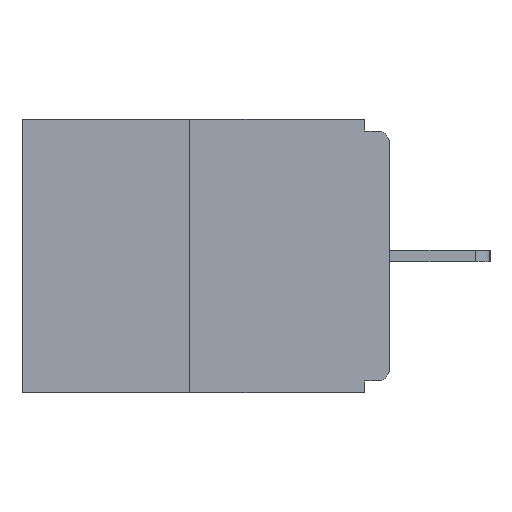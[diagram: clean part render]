
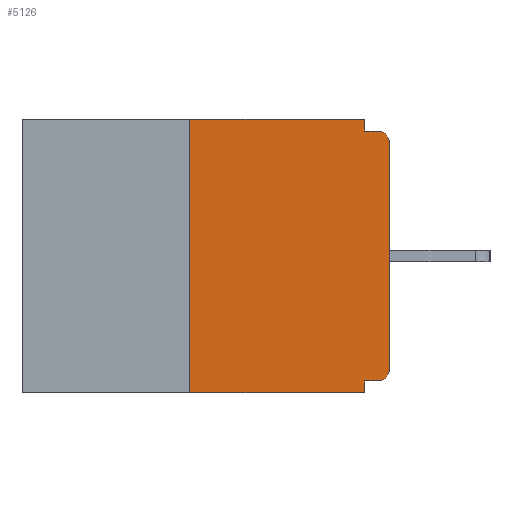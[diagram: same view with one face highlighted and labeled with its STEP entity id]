
A CAD part, left-side view. The second image highlights one B-rep face of the part: STEP entity #5126.
In plain terms, the highlighted planar face has unit normal (-1, 0, 0).
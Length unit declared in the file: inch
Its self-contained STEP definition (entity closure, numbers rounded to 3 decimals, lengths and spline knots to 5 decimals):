
#54 = CARTESIAN_POINT ( 'NONE',  ( 0., 0.031, -0.328 ) ) ;
#58 = ORIENTED_EDGE ( 'NONE', *, *, #1435, .F. ) ;
#370 = VECTOR ( 'NONE', #8513, 39.37008 ) ;
#512 = DIRECTION ( 'NONE',  ( 0., 1., 0. ) ) ;
#694 = CARTESIAN_POINT ( 'NONE',  ( 0., 0.031, -0.343 ) ) ;
#1266 = LINE ( 'NONE', #2451, #4930 ) ;
#1435 = EDGE_CURVE ( 'NONE', #9953, #11994, #3227, .T. ) ;
#1493 = DIRECTION ( 'NONE',  ( -1., 0., 0. ) ) ;
#1563 = EDGE_CURVE ( 'NONE', #3779, #13840, #5796, .T. ) ;
#2316 = DIRECTION ( 'NONE',  ( -1., 0., 0. ) ) ;
#2371 = LINE ( 'NONE', #694, #10799 ) ;
#2451 = CARTESIAN_POINT ( 'NONE',  ( 0., 0.25, 0. ) ) ;
#2717 = VERTEX_POINT ( 'NONE', #14361 ) ;
#2889 = CIRCLE ( 'NONE', #16332, 0.015 ) ;
#3047 = ORIENTED_EDGE ( 'NONE', *, *, #3152, .T. ) ;
#3152 = EDGE_CURVE ( 'NONE', #7802, #6265, #6615, .T. ) ;
#3227 = LINE ( 'NONE', #5793, #6926 ) ;
#3363 = CARTESIAN_POINT ( 'NONE',  ( 0., 0.25, 0. ) ) ;
#3403 = ORIENTED_EDGE ( 'NONE', *, *, #1563, .F. ) ;
#3779 = VERTEX_POINT ( 'NONE', #4391 ) ;
#3789 = EDGE_CURVE ( 'NONE', #8034, #10893, #13545, .T. ) ;
#3894 = CIRCLE ( 'NONE', #10600, 0.015 ) ;
#3910 = VERTEX_POINT ( 'NONE', #12890 ) ;
#4391 = CARTESIAN_POINT ( 'NONE',  ( 0., 0.015, -0.328 ) ) ;
#4912 = DIRECTION ( 'NONE',  ( 0., 0., -1. ) ) ;
#4930 = VECTOR ( 'NONE', #16602, 39.37008 ) ;
#5126 = ADVANCED_FACE ( 'NONE', ( #14626 ), #14539, .F. ) ;
#5397 = ORIENTED_EDGE ( 'NONE', *, *, #14566, .F. ) ;
#5653 = CARTESIAN_POINT ( 'NONE',  ( 0., 0.015, -0.015 ) ) ;
#5793 = CARTESIAN_POINT ( 'NONE',  ( 0., 0.46, 0. ) ) ;
#5796 = LINE ( 'NONE', #12034, #15717 ) ;
#5838 = ORIENTED_EDGE ( 'NONE', *, *, #3789, .F. ) ;
#6115 = CARTESIAN_POINT ( 'NONE',  ( 0., 0.25, -0.343 ) ) ;
#6218 = EDGE_CURVE ( 'NONE', #3779, #2717, #2889, .T. ) ;
#6265 = VERTEX_POINT ( 'NONE', #9070 ) ;
#6615 = LINE ( 'NONE', #10829, #9888 ) ;
#6686 = CARTESIAN_POINT ( 'NONE',  ( 0., 0., 0. ) ) ;
#6926 = VECTOR ( 'NONE', #10938, 39.37008 ) ;
#7516 = CARTESIAN_POINT ( 'NONE',  ( 0., 0.015, -0.03 ) ) ;
#7526 = EDGE_LOOP ( 'NONE', ( #58, #11486, #3047, #12841, #3403, #14533, #8023, #10892, #5838, #5397 ) ) ;
#7571 = DIRECTION ( 'NONE',  ( 0., 0., -1. ) ) ;
#7802 = VERTEX_POINT ( 'NONE', #6115 ) ;
#7807 = DIRECTION ( 'NONE',  ( 0., 0., -1. ) ) ;
#7978 = DIRECTION ( 'NONE',  ( 0., -1., 0. ) ) ;
#8023 = ORIENTED_EDGE ( 'NONE', *, *, #10318, .T. ) ;
#8034 = VERTEX_POINT ( 'NONE', #9715 ) ;
#8156 = CARTESIAN_POINT ( 'NONE',  ( 0., 0., -0.015 ) ) ;
#8330 = DIRECTION ( 'NONE',  ( 0., -1., 0. ) ) ;
#8513 = DIRECTION ( 'NONE',  ( 0., 0., -1. ) ) ;
#9070 = CARTESIAN_POINT ( 'NONE',  ( 0., 0.031, -0.343 ) ) ;
#9715 = CARTESIAN_POINT ( 'NONE',  ( 0., 0.031, -0.015 ) ) ;
#9860 = CARTESIAN_POINT ( 'NONE',  ( 0., 0.031, 0. ) ) ;
#9888 = VECTOR ( 'NONE', #7978, 39.37008 ) ;
#9953 = VERTEX_POINT ( 'NONE', #3363 ) ;
#10318 = EDGE_CURVE ( 'NONE', #2717, #3910, #13024, .T. ) ;
#10600 = AXIS2_PLACEMENT_3D ( 'NONE', #7516, #2316, #4912 ) ;
#10799 = VECTOR ( 'NONE', #7571, 39.37008 ) ;
#10829 = CARTESIAN_POINT ( 'NONE',  ( 0., 0.46, -0.343 ) ) ;
#10892 = ORIENTED_EDGE ( 'NONE', *, *, #15446, .T. ) ;
#10893 = VERTEX_POINT ( 'NONE', #5653 ) ;
#10938 = DIRECTION ( 'NONE',  ( 0., -1., 0. ) ) ;
#10941 = EDGE_CURVE ( 'NONE', #13840, #6265, #2371, .T. ) ;
#11486 = ORIENTED_EDGE ( 'NONE', *, *, #14748, .F. ) ;
#11587 = VECTOR ( 'NONE', #11831, 39.37008 ) ;
#11831 = DIRECTION ( 'NONE',  ( 0., 0., 1. ) ) ;
#11994 = VERTEX_POINT ( 'NONE', #15461 ) ;
#11995 = DIRECTION ( 'NONE',  ( 0., 0., -1. ) ) ;
#12034 = CARTESIAN_POINT ( 'NONE',  ( 0., 0., -0.328 ) ) ;
#12274 = AXIS2_PLACEMENT_3D ( 'NONE', #15806, #13349, #11995 ) ;
#12384 = LINE ( 'NONE', #9860, #370 ) ;
#12841 = ORIENTED_EDGE ( 'NONE', *, *, #10941, .F. ) ;
#12890 = CARTESIAN_POINT ( 'NONE',  ( 0., 0., -0.03 ) ) ;
#13024 = LINE ( 'NONE', #6686, #11587 ) ;
#13349 = DIRECTION ( 'NONE',  ( 1., 0., 0. ) ) ;
#13545 = LINE ( 'NONE', #8156, #14913 ) ;
#13840 = VERTEX_POINT ( 'NONE', #54 ) ;
#14361 = CARTESIAN_POINT ( 'NONE',  ( 0., 0., -0.313 ) ) ;
#14368 = CARTESIAN_POINT ( 'NONE',  ( 0., 0.015, -0.313 ) ) ;
#14533 = ORIENTED_EDGE ( 'NONE', *, *, #6218, .T. ) ;
#14539 = PLANE ( 'NONE',  #12274 ) ;
#14566 = EDGE_CURVE ( 'NONE', #11994, #8034, #12384, .T. ) ;
#14626 = FACE_OUTER_BOUND ( 'NONE', #7526, .T. ) ;
#14748 = EDGE_CURVE ( 'NONE', #7802, #9953, #1266, .T. ) ;
#14913 = VECTOR ( 'NONE', #8330, 39.37008 ) ;
#15446 = EDGE_CURVE ( 'NONE', #3910, #10893, #3894, .T. ) ;
#15461 = CARTESIAN_POINT ( 'NONE',  ( 0., 0.031, 0. ) ) ;
#15717 = VECTOR ( 'NONE', #512, 39.37008 ) ;
#15806 = CARTESIAN_POINT ( 'NONE',  ( 0., 0.46, 0. ) ) ;
#16332 = AXIS2_PLACEMENT_3D ( 'NONE', #14368, #1493, #7807 ) ;
#16602 = DIRECTION ( 'NONE',  ( 0., 0., 1. ) ) ;
